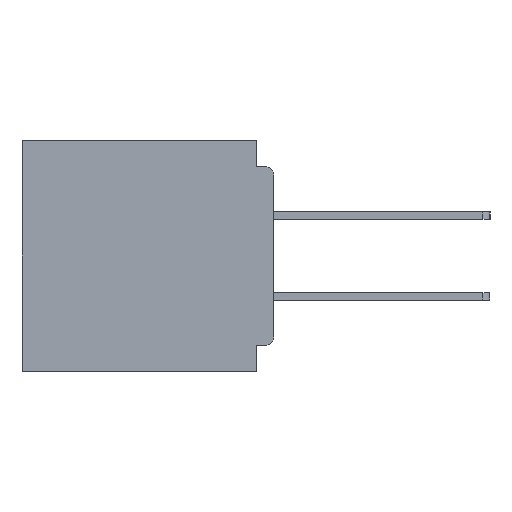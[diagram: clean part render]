
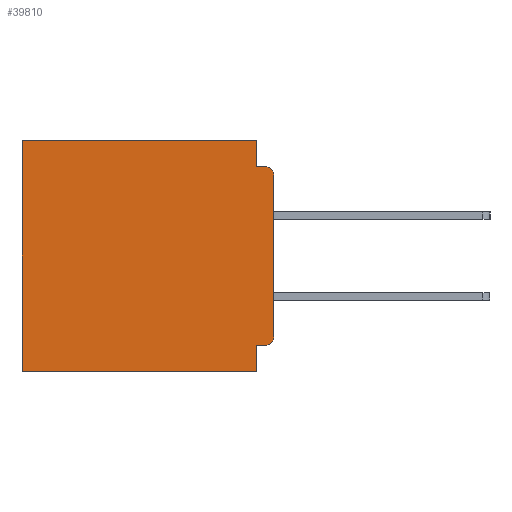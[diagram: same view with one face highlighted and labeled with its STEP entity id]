
A CAD part, left-side view. The second image highlights one B-rep face of the part: STEP entity #39810.
In plain terms, the highlighted planar face has unit normal (-1, 0, 0).
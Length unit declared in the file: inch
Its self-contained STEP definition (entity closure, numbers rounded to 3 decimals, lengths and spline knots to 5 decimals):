
#873 = CARTESIAN_POINT ( 'NONE',  ( 0.3, 0., -0.4 ) ) ;
#1321 = LINE ( 'NONE', #14877, #8448 ) ;
#2074 = ORIENTED_EDGE ( 'NONE', *, *, #3624, .F. ) ;
#2114 = EDGE_CURVE ( 'NONE', #29407, #6334, #6711, .T. ) ;
#3624 = EDGE_CURVE ( 'NONE', #50006, #33998, #1321, .T. ) ;
#3925 = VECTOR ( 'NONE', #42726, 39.37008 ) ;
#4526 = AXIS2_PLACEMENT_3D ( 'NONE', #873, #33851, #9389 ) ;
#5474 = EDGE_CURVE ( 'NONE', #26144, #50006, #30759, .T. ) ;
#6334 = VERTEX_POINT ( 'NONE', #18058 ) ;
#6711 = LINE ( 'NONE', #22710, #15037 ) ;
#6946 = DIRECTION ( 'NONE',  ( -1., 0., 0. ) ) ;
#7822 = EDGE_LOOP ( 'NONE', ( #45989, #7892, #2074, #13066, #34821, #47399, #10594, #20832, #30517, #33064 ) ) ;
#7892 = ORIENTED_EDGE ( 'NONE', *, *, #36668, .T. ) ;
#8448 = VECTOR ( 'NONE', #26871, 39.37008 ) ;
#8955 = AXIS2_PLACEMENT_3D ( 'NONE', #47902, #23709, #51925 ) ;
#9389 = DIRECTION ( 'NONE',  ( 0., 0., -1. ) ) ;
#9731 = CARTESIAN_POINT ( 'NONE',  ( 0.3, 0.437, -0.4 ) ) ;
#10188 = CARTESIAN_POINT ( 'NONE',  ( 0.3, 0., -0.4 ) ) ;
#10594 = ORIENTED_EDGE ( 'NONE', *, *, #25228, .F. ) ;
#12264 = EDGE_CURVE ( 'NONE', #34360, #45073, #28825, .T. ) ;
#12694 = LINE ( 'NONE', #14673, #20957 ) ;
#13014 = EDGE_CURVE ( 'NONE', #26144, #34297, #13367, .T. ) ;
#13066 = ORIENTED_EDGE ( 'NONE', *, *, #5474, .F. ) ;
#13367 = LINE ( 'NONE', #32253, #22943 ) ;
#14673 = CARTESIAN_POINT ( 'NONE',  ( 0.3, 0., -0.355 ) ) ;
#14877 = CARTESIAN_POINT ( 'NONE',  ( 0.3, 0., -0.045 ) ) ;
#15037 = VECTOR ( 'NONE', #23961, 39.37008 ) ;
#15311 = DIRECTION ( 'NONE',  ( 0., 0., -1. ) ) ;
#15420 = DIRECTION ( 'NONE',  ( 0., 0., -1. ) ) ;
#15965 = DIRECTION ( 'NONE',  ( 0., 1., 0. ) ) ;
#16535 = CARTESIAN_POINT ( 'NONE',  ( 0.3, 0.031, 0. ) ) ;
#18058 = CARTESIAN_POINT ( 'NONE',  ( 0.3, 0.031, -0.4 ) ) ;
#18596 = CARTESIAN_POINT ( 'NONE',  ( 0.3, 0.015, -0.045 ) ) ;
#18766 = DIRECTION ( 'NONE',  ( 0., 1., 0. ) ) ;
#19856 = VECTOR ( 'NONE', #24744, 39.37008 ) ;
#20832 = ORIENTED_EDGE ( 'NONE', *, *, #2114, .F. ) ;
#20842 = EDGE_CURVE ( 'NONE', #34297, #38060, #36583, .T. ) ;
#20957 = VECTOR ( 'NONE', #18766, 39.37008 ) ;
#21030 = CARTESIAN_POINT ( 'NONE',  ( 0.3, 0.015, -0.355 ) ) ;
#22710 = CARTESIAN_POINT ( 'NONE',  ( 0.3, 0.031, -0.4 ) ) ;
#22943 = VECTOR ( 'NONE', #15965, 39.37008 ) ;
#23470 = EDGE_CURVE ( 'NONE', #34360, #29407, #12694, .T. ) ;
#23709 = DIRECTION ( 'NONE',  ( -1., 0., 0. ) ) ;
#23961 = DIRECTION ( 'NONE',  ( 0., 0., -1. ) ) ;
#24744 = DIRECTION ( 'NONE',  ( 0., 0., -1. ) ) ;
#25228 = EDGE_CURVE ( 'NONE', #6334, #38060, #36502, .T. ) ;
#25732 = VECTOR ( 'NONE', #15311, 39.37008 ) ;
#26144 = VERTEX_POINT ( 'NONE', #39268 ) ;
#26721 = AXIS2_PLACEMENT_3D ( 'NONE', #31480, #6946, #35526 ) ;
#26871 = DIRECTION ( 'NONE',  ( 0., -1., 0. ) ) ;
#27422 = CARTESIAN_POINT ( 'NONE',  ( 0.3, 0.031, -0.045 ) ) ;
#28825 = CIRCLE ( 'NONE', #8955, 0.015 ) ;
#29407 = VERTEX_POINT ( 'NONE', #33525 ) ;
#30517 = ORIENTED_EDGE ( 'NONE', *, *, #23470, .F. ) ;
#30759 = LINE ( 'NONE', #16535, #19856 ) ;
#31480 = CARTESIAN_POINT ( 'NONE',  ( 0.3, 0.015, -0.06 ) ) ;
#31708 = LINE ( 'NONE', #39793, #41109 ) ;
#32253 = CARTESIAN_POINT ( 'NONE',  ( 0.3, 0., 0. ) ) ;
#32695 = CARTESIAN_POINT ( 'NONE',  ( 0.3, 0.437, 0. ) ) ;
#33064 = ORIENTED_EDGE ( 'NONE', *, *, #12264, .T. ) ;
#33525 = CARTESIAN_POINT ( 'NONE',  ( 0.3, 0.031, -0.355 ) ) ;
#33851 = DIRECTION ( 'NONE',  ( 1., 0., 0. ) ) ;
#33998 = VERTEX_POINT ( 'NONE', #18596 ) ;
#34297 = VERTEX_POINT ( 'NONE', #32695 ) ;
#34360 = VERTEX_POINT ( 'NONE', #21030 ) ;
#34821 = ORIENTED_EDGE ( 'NONE', *, *, #13014, .T. ) ;
#35368 = CARTESIAN_POINT ( 'NONE',  ( 0.3, 0., -0.34 ) ) ;
#35526 = DIRECTION ( 'NONE',  ( 0., 0., -1. ) ) ;
#36502 = LINE ( 'NONE', #10188, #3925 ) ;
#36583 = LINE ( 'NONE', #43521, #25732 ) ;
#36668 = EDGE_CURVE ( 'NONE', #45493, #33998, #48611, .T. ) ;
#38060 = VERTEX_POINT ( 'NONE', #9731 ) ;
#38135 = CARTESIAN_POINT ( 'NONE',  ( 0.3, 0., -0.06 ) ) ;
#38804 = EDGE_CURVE ( 'NONE', #45493, #45073, #31708, .T. ) ;
#39268 = CARTESIAN_POINT ( 'NONE',  ( 0.3, 0.031, 0. ) ) ;
#39793 = CARTESIAN_POINT ( 'NONE',  ( 0.3, 0., -0.4 ) ) ;
#39810 = ADVANCED_FACE ( 'NONE', ( #46630 ), #49796, .F. ) ;
#41109 = VECTOR ( 'NONE', #15420, 39.37008 ) ;
#42726 = DIRECTION ( 'NONE',  ( 0., 1., 0. ) ) ;
#43521 = CARTESIAN_POINT ( 'NONE',  ( 0.3, 0.437, -0.4 ) ) ;
#45073 = VERTEX_POINT ( 'NONE', #35368 ) ;
#45493 = VERTEX_POINT ( 'NONE', #38135 ) ;
#45989 = ORIENTED_EDGE ( 'NONE', *, *, #38804, .F. ) ;
#46630 = FACE_OUTER_BOUND ( 'NONE', #7822, .T. ) ;
#47399 = ORIENTED_EDGE ( 'NONE', *, *, #20842, .T. ) ;
#47902 = CARTESIAN_POINT ( 'NONE',  ( 0.3, 0.015, -0.34 ) ) ;
#48611 = CIRCLE ( 'NONE', #26721, 0.015 ) ;
#49796 = PLANE ( 'NONE',  #4526 ) ;
#50006 = VERTEX_POINT ( 'NONE', #27422 ) ;
#51925 = DIRECTION ( 'NONE',  ( 0., 0., -1. ) ) ;
